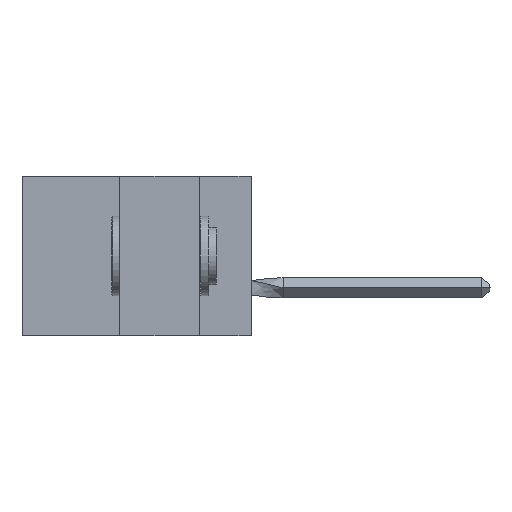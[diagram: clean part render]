
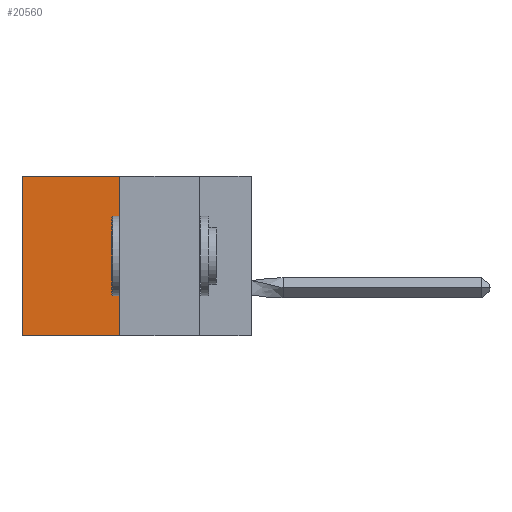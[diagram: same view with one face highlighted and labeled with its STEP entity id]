
A CAD part, left-side view. The second image highlights one B-rep face of the part: STEP entity #20560.
In plain terms, the highlighted planar face has unit normal (-1, 0, 0).
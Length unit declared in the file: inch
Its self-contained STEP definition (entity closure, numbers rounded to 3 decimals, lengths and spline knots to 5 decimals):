
#1243 = CARTESIAN_POINT ( 'NONE',  ( 0.305, 0.72, -0.5 ) ) ;
#3225 = LINE ( 'NONE', #16107, #5391 ) ;
#3585 = LINE ( 'NONE', #9777, #21120 ) ;
#3845 = VERTEX_POINT ( 'NONE', #14466 ) ;
#3912 = AXIS2_PLACEMENT_3D ( 'NONE', #16516, #6171, #13073 ) ;
#3961 = EDGE_CURVE ( 'NONE', #10786, #3845, #14711, .T. ) ;
#4913 = EDGE_CURVE ( 'NONE', #7181, #10786, #3225, .T. ) ;
#4989 = LINE ( 'NONE', #12654, #5529 ) ;
#5167 = CARTESIAN_POINT ( 'NONE',  ( 0.305, 0.72, 0. ) ) ;
#5391 = VECTOR ( 'NONE', #7617, 39.37008 ) ;
#5529 = VECTOR ( 'NONE', #21124, 39.37008 ) ;
#6171 = DIRECTION ( 'NONE',  ( 1., 0., 0. ) ) ;
#7181 = VERTEX_POINT ( 'NONE', #9433 ) ;
#7617 = DIRECTION ( 'NONE',  ( 0., 1., 0. ) ) ;
#8701 = EDGE_CURVE ( 'NONE', #7181, #11917, #4989, .T. ) ;
#9433 = CARTESIAN_POINT ( 'NONE',  ( 0.305, 0.413, 0. ) ) ;
#9640 = PLANE ( 'NONE',  #3912 ) ;
#9777 = CARTESIAN_POINT ( 'NONE',  ( 0.305, 0.413, -0.5 ) ) ;
#10786 = VERTEX_POINT ( 'NONE', #5167 ) ;
#11204 = EDGE_CURVE ( 'NONE', #11917, #3845, #3585, .T. ) ;
#11610 = DIRECTION ( 'NONE',  ( 0., 0., -1. ) ) ;
#11917 = VERTEX_POINT ( 'NONE', #16154 ) ;
#12622 = ORIENTED_EDGE ( 'NONE', *, *, #3961, .T. ) ;
#12654 = CARTESIAN_POINT ( 'NONE',  ( 0.305, 0.413, -0.5 ) ) ;
#13073 = DIRECTION ( 'NONE',  ( 0., 0., -1. ) ) ;
#13248 = EDGE_LOOP ( 'NONE', ( #12622, #18965, #21988, #19812 ) ) ;
#14466 = CARTESIAN_POINT ( 'NONE',  ( 0.305, 0.72, -0.5 ) ) ;
#14711 = LINE ( 'NONE', #1243, #19763 ) ;
#16107 = CARTESIAN_POINT ( 'NONE',  ( 0.305, 0.413, 0. ) ) ;
#16154 = CARTESIAN_POINT ( 'NONE',  ( 0.305, 0.413, -0.5 ) ) ;
#16516 = CARTESIAN_POINT ( 'NONE',  ( 0.305, 0.413, -0.5 ) ) ;
#16583 = DIRECTION ( 'NONE',  ( 0., 1., 0. ) ) ;
#18965 = ORIENTED_EDGE ( 'NONE', *, *, #11204, .F. ) ;
#19763 = VECTOR ( 'NONE', #11610, 39.37008 ) ;
#19812 = ORIENTED_EDGE ( 'NONE', *, *, #4913, .T. ) ;
#20560 = ADVANCED_FACE ( 'NONE', ( #20764 ), #9640, .F. ) ;
#20764 = FACE_OUTER_BOUND ( 'NONE', #13248, .T. ) ;
#21120 = VECTOR ( 'NONE', #16583, 39.37008 ) ;
#21124 = DIRECTION ( 'NONE',  ( 0., 0., -1. ) ) ;
#21988 = ORIENTED_EDGE ( 'NONE', *, *, #8701, .F. ) ;
